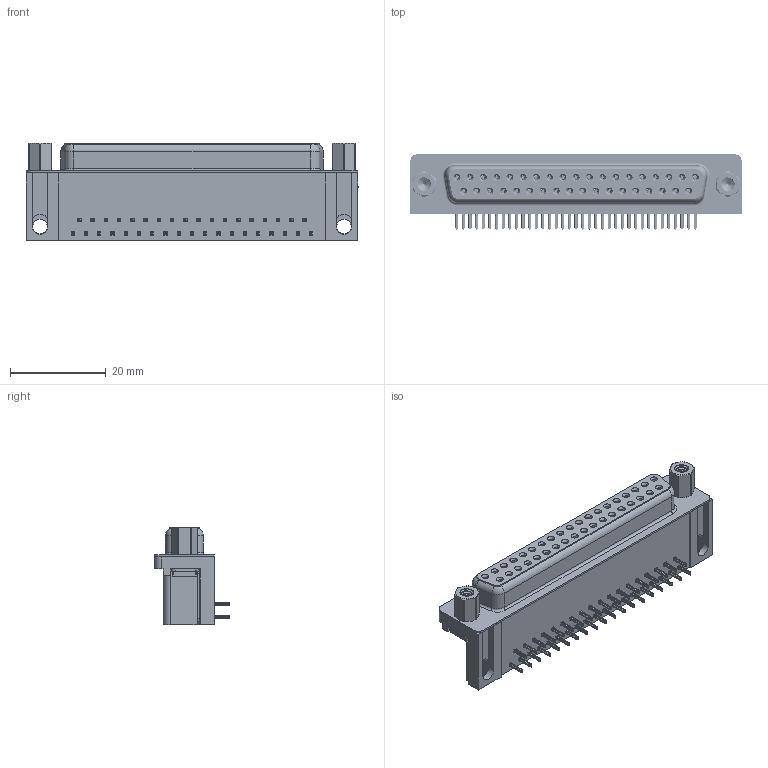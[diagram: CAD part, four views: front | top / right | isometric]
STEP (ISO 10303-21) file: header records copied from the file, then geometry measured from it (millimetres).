
FILE_DESCRIPTION (( 'STEP AP203' ), '1' );
FILE_NAME ('630-037-640-013.STEP', '2021-09-22T14:33:38', ( '' ), ( '' ), 'SwSTEP 2.0', 'SolidWorks 2020', '' );
FILE_SCHEMA (( 'CONFIG_CONTROL_DESIGN' ));
Length unit declared in the file: millimetre
Products named in the file (8): 630 Housing_37 Socket; 630 Thru Hole Board Mount; 630 Shell_37 Socket; 630-037-640-013; 630 4-40 Threaded Rivet; 630 4-40 Hex Standoff 5; 630 Contact Top; 630 Contact Bottom
Assembly tree (45 placements, depth 2):
  630-037-640-013
    630 Housing_37 Socket
    630 Shell_37 Socket
    630 Contact Bottom  x18
    630 Contact Top  x19
    630 Thru Hole Board Mount  x2
    630 4-40 Threaded Rivet  x2
    630 4-40 Hex Standoff 5  x2
Bounding box: 69.4 x 15.73 x 20.4 mm (x, y, z)
Volume: 12026.8 mm3; surface area: 14017.5 mm2
Topology: 45 solids, 45 shells, 5686 faces, 14940 edges, 9370 vertices
Faces by surface type: plane 2524, cylinder 1370, bspline 1278, cone 476, torus 38
Entity records: 41015 total; most frequent: CARTESIAN_POINT 13801, ORIENTED_EDGE 5372, DIRECTION 4967, EDGE_CURVE 2686, LINE 1753, VECTOR 1753, VERTEX_POINT 1721, AXIS2_PLACEMENT_3D 1607
